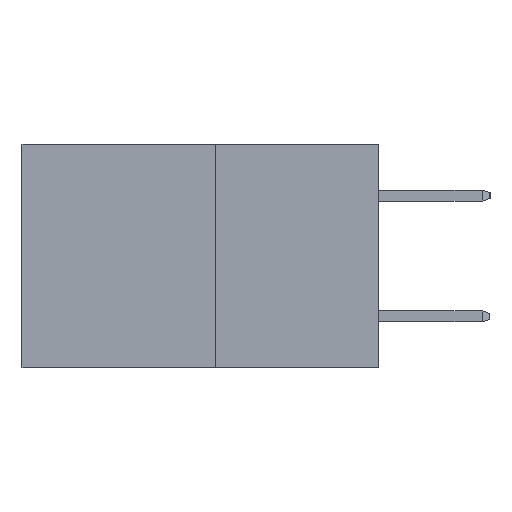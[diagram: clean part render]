
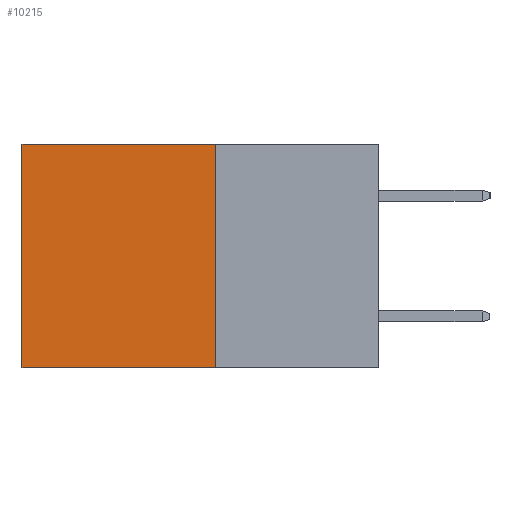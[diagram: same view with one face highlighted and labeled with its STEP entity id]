
A CAD part, left-side view. The second image highlights one B-rep face of the part: STEP entity #10215.
In plain terms, the highlighted planar face has unit normal (-1, 0, 0).
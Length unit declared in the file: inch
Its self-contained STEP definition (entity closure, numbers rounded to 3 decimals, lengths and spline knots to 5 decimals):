
#166 = VERTEX_POINT ( 'NONE', #3091 ) ;
#317 = DIRECTION ( 'NONE',  ( 0., 0., -1. ) ) ;
#863 = LINE ( 'NONE', #9219, #8121 ) ;
#1001 = EDGE_CURVE ( 'NONE', #7564, #6240, #11705, .T. ) ;
#1621 = VECTOR ( 'NONE', #9838, 39.37008 ) ;
#2373 = CARTESIAN_POINT ( 'NONE',  ( 0.277, 0.27, 0. ) ) ;
#2769 = ORIENTED_EDGE ( 'NONE', *, *, #6156, .T. ) ;
#2774 = CARTESIAN_POINT ( 'NONE',  ( 0.277, 0.27, 0. ) ) ;
#2894 = ORIENTED_EDGE ( 'NONE', *, *, #5092, .F. ) ;
#3016 = ORIENTED_EDGE ( 'NONE', *, *, #4298, .F. ) ;
#3043 = ORIENTED_EDGE ( 'NONE', *, *, #1001, .T. ) ;
#3051 = CARTESIAN_POINT ( 'NONE',  ( 0.277, 0.27, -0.37 ) ) ;
#3091 = CARTESIAN_POINT ( 'NONE',  ( 0.277, 0.59, -0.37 ) ) ;
#3361 = DIRECTION ( 'NONE',  ( 0., 0., -1. ) ) ;
#4277 = VECTOR ( 'NONE', #3361, 39.37008 ) ;
#4298 = EDGE_CURVE ( 'NONE', #7564, #11183, #9337, .T. ) ;
#4872 = EDGE_LOOP ( 'NONE', ( #2769, #2894, #3016, #3043 ) ) ;
#5092 = EDGE_CURVE ( 'NONE', #11183, #166, #8300, .T. ) ;
#5670 = FACE_OUTER_BOUND ( 'NONE', #4872, .T. ) ;
#6156 = EDGE_CURVE ( 'NONE', #6240, #166, #863, .T. ) ;
#6240 = VERTEX_POINT ( 'NONE', #10949 ) ;
#6325 = DIRECTION ( 'NONE',  ( 1., 0., 0. ) ) ;
#6603 = AXIS2_PLACEMENT_3D ( 'NONE', #12082, #6325, #317 ) ;
#7564 = VERTEX_POINT ( 'NONE', #2373 ) ;
#8121 = VECTOR ( 'NONE', #11333, 39.37008 ) ;
#8300 = LINE ( 'NONE', #12559, #10552 ) ;
#9017 = CARTESIAN_POINT ( 'NONE',  ( 0.277, 0.27, -0.37 ) ) ;
#9219 = CARTESIAN_POINT ( 'NONE',  ( 0.277, 0.59, -0.37 ) ) ;
#9337 = LINE ( 'NONE', #3051, #4277 ) ;
#9838 = DIRECTION ( 'NONE',  ( 0., 1., 0. ) ) ;
#10215 = ADVANCED_FACE ( 'NONE', ( #5670 ), #11112, .F. ) ;
#10552 = VECTOR ( 'NONE', #12507, 39.37008 ) ;
#10949 = CARTESIAN_POINT ( 'NONE',  ( 0.277, 0.59, 0. ) ) ;
#11112 = PLANE ( 'NONE',  #6603 ) ;
#11183 = VERTEX_POINT ( 'NONE', #9017 ) ;
#11333 = DIRECTION ( 'NONE',  ( 0., 0., -1. ) ) ;
#11705 = LINE ( 'NONE', #2774, #1621 ) ;
#12082 = CARTESIAN_POINT ( 'NONE',  ( 0.277, 0.27, -0.37 ) ) ;
#12507 = DIRECTION ( 'NONE',  ( 0., 1., 0. ) ) ;
#12559 = CARTESIAN_POINT ( 'NONE',  ( 0.277, 0.27, -0.37 ) ) ;
